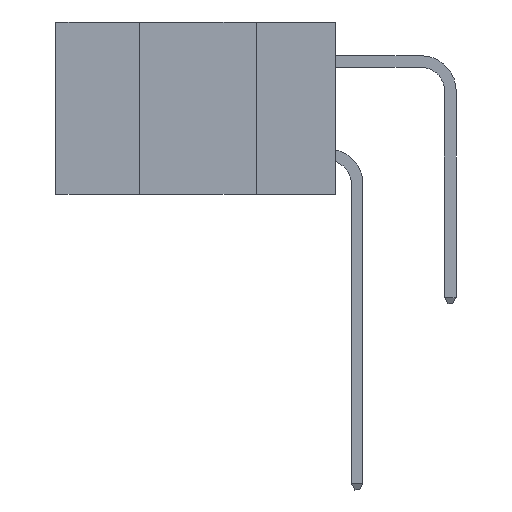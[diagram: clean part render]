
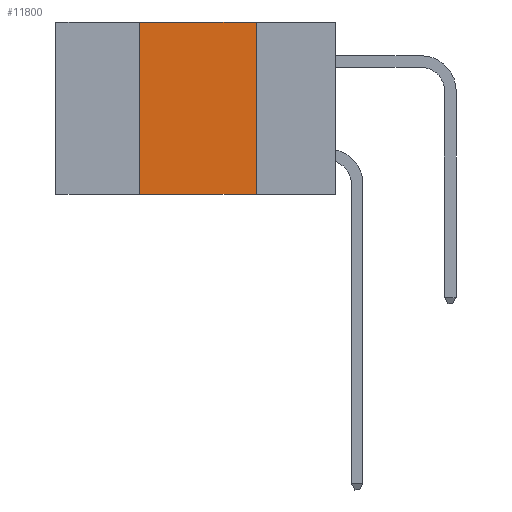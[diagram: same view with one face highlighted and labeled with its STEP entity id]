
A CAD part, left-side view. The second image highlights one B-rep face of the part: STEP entity #11800.
In plain terms, the highlighted planar face has unit normal (-1, 0, 0).
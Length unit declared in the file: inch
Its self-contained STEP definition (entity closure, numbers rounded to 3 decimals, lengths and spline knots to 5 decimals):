
#455 = VECTOR ( 'NONE', #17929, 39.37008 ) ;
#781 = ORIENTED_EDGE ( 'NONE', *, *, #3638, .F. ) ;
#1234 = DIRECTION ( 'NONE',  ( 0., 0., -1. ) ) ;
#1397 = VECTOR ( 'NONE', #13114, 39.37008 ) ;
#2618 = DIRECTION ( 'NONE',  ( 0., -1., 0. ) ) ;
#2662 = DIRECTION ( 'NONE',  ( 1., 0., 0. ) ) ;
#3050 = CARTESIAN_POINT ( 'NONE',  ( 0., 0.17, -0.37 ) ) ;
#3638 = EDGE_CURVE ( 'NONE', #16879, #7846, #18892, .T. ) ;
#3813 = VERTEX_POINT ( 'NONE', #3050 ) ;
#4224 = VERTEX_POINT ( 'NONE', #5646 ) ;
#5124 = FACE_OUTER_BOUND ( 'NONE', #16442, .T. ) ;
#5523 = CARTESIAN_POINT ( 'NONE',  ( 0., 0.6, 0. ) ) ;
#5646 = CARTESIAN_POINT ( 'NONE',  ( 0., 0.17, 0. ) ) ;
#6095 = VECTOR ( 'NONE', #14872, 39.37008 ) ;
#6297 = CARTESIAN_POINT ( 'NONE',  ( 0., 0.42, 0. ) ) ;
#7846 = VERTEX_POINT ( 'NONE', #6297 ) ;
#8340 = LINE ( 'NONE', #8963, #455 ) ;
#8480 = PLANE ( 'NONE',  #10016 ) ;
#8623 = LINE ( 'NONE', #10575, #6095 ) ;
#8963 = CARTESIAN_POINT ( 'NONE',  ( 0., 0.17, 0. ) ) ;
#10016 = AXIS2_PLACEMENT_3D ( 'NONE', #5523, #2662, #1234 ) ;
#10390 = EDGE_CURVE ( 'NONE', #16879, #3813, #17145, .T. ) ;
#10541 = ORIENTED_EDGE ( 'NONE', *, *, #10390, .T. ) ;
#10575 = CARTESIAN_POINT ( 'NONE',  ( 0., 0.6, 0. ) ) ;
#10974 = EDGE_CURVE ( 'NONE', #7846, #4224, #8623, .T. ) ;
#11800 = ADVANCED_FACE ( 'NONE', ( #5124 ), #8480, .F. ) ;
#13114 = DIRECTION ( 'NONE',  ( 0., 0., 1. ) ) ;
#13519 = ORIENTED_EDGE ( 'NONE', *, *, #10974, .F. ) ;
#14489 = CARTESIAN_POINT ( 'NONE',  ( 0., 0.42, 0. ) ) ;
#14872 = DIRECTION ( 'NONE',  ( 0., -1., 0. ) ) ;
#16442 = EDGE_LOOP ( 'NONE', ( #16696, #13519, #781, #10541 ) ) ;
#16493 = EDGE_CURVE ( 'NONE', #4224, #3813, #8340, .T. ) ;
#16696 = ORIENTED_EDGE ( 'NONE', *, *, #16493, .F. ) ;
#16879 = VERTEX_POINT ( 'NONE', #18506 ) ;
#17145 = LINE ( 'NONE', #18763, #18518 ) ;
#17929 = DIRECTION ( 'NONE',  ( 0., 0., -1. ) ) ;
#18506 = CARTESIAN_POINT ( 'NONE',  ( 0., 0.42, -0.37 ) ) ;
#18518 = VECTOR ( 'NONE', #2618, 39.37008 ) ;
#18763 = CARTESIAN_POINT ( 'NONE',  ( 0., 0.6, -0.37 ) ) ;
#18892 = LINE ( 'NONE', #14489, #1397 ) ;
